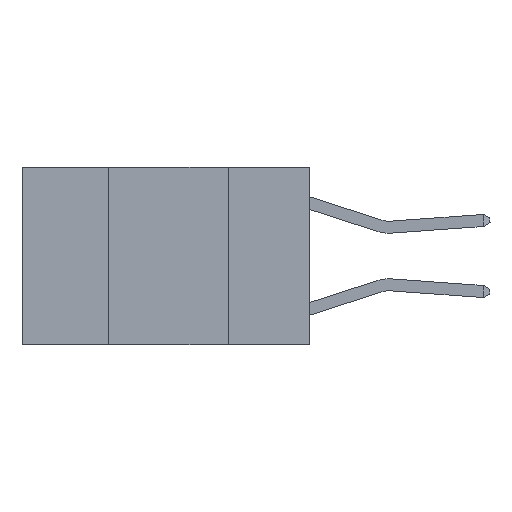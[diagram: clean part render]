
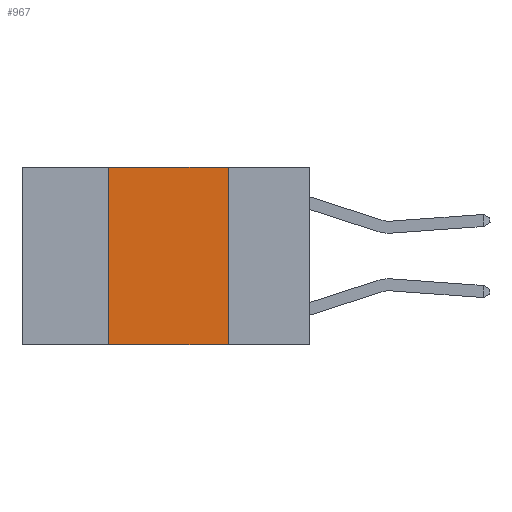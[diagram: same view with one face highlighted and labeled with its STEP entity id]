
A CAD part, left-side view. The second image highlights one B-rep face of the part: STEP entity #967.
In plain terms, the highlighted planar face has unit normal (-1, 0, 0).
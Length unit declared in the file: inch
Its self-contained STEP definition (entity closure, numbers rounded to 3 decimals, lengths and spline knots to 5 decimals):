
#78 = ORIENTED_EDGE ( 'NONE', *, *, #5642, .F. ) ;
#271 = ORIENTED_EDGE ( 'NONE', *, *, #17563, .F. ) ;
#313 = ORIENTED_EDGE ( 'NONE', *, *, #11521, .F. ) ;
#607 = PLANE ( 'NONE',  #19080 ) ;
#947 = ORIENTED_EDGE ( 'NONE', *, *, #10591, .T. ) ;
#967 = ADVANCED_FACE ( 'NONE', ( #11820 ), #607, .F. ) ;
#1670 = VERTEX_POINT ( 'NONE', #7644 ) ;
#1758 = CARTESIAN_POINT ( 'NONE',  ( 0., 0.42, -0.37 ) ) ;
#2449 = VECTOR ( 'NONE', #8322, 39.37008 ) ;
#2962 = VERTEX_POINT ( 'NONE', #1758 ) ;
#5642 = EDGE_CURVE ( 'NONE', #1670, #18077, #13989, .T. ) ;
#6586 = DIRECTION ( 'NONE',  ( 0., 0., -1. ) ) ;
#7082 = CARTESIAN_POINT ( 'NONE',  ( 0., 0.42, 0. ) ) ;
#7644 = CARTESIAN_POINT ( 'NONE',  ( 0., 0.17, 0. ) ) ;
#7952 = DIRECTION ( 'NONE',  ( 0., -1., 0. ) ) ;
#8322 = DIRECTION ( 'NONE',  ( 0., 0., -1. ) ) ;
#8584 = DIRECTION ( 'NONE',  ( 0., 0., 1. ) ) ;
#9058 = VECTOR ( 'NONE', #7952, 39.37008 ) ;
#9167 = VECTOR ( 'NONE', #15665, 39.37008 ) ;
#9827 = VERTEX_POINT ( 'NONE', #19025 ) ;
#10449 = DIRECTION ( 'NONE',  ( 1., 0., 0. ) ) ;
#10591 = EDGE_CURVE ( 'NONE', #2962, #18077, #17061, .T. ) ;
#11521 = EDGE_CURVE ( 'NONE', #2962, #9827, #14922, .T. ) ;
#11820 = FACE_OUTER_BOUND ( 'NONE', #14012, .T. ) ;
#12239 = CARTESIAN_POINT ( 'NONE',  ( 0., 0.17, -0.37 ) ) ;
#12422 = CARTESIAN_POINT ( 'NONE',  ( 0., 0.6, -0.37 ) ) ;
#13151 = LINE ( 'NONE', #18550, #9167 ) ;
#13989 = LINE ( 'NONE', #18808, #2449 ) ;
#14012 = EDGE_LOOP ( 'NONE', ( #78, #271, #313, #947 ) ) ;
#14447 = VECTOR ( 'NONE', #8584, 39.37008 ) ;
#14922 = LINE ( 'NONE', #7082, #14447 ) ;
#15665 = DIRECTION ( 'NONE',  ( 0., -1., 0. ) ) ;
#17061 = LINE ( 'NONE', #12422, #9058 ) ;
#17563 = EDGE_CURVE ( 'NONE', #9827, #1670, #13151, .T. ) ;
#18077 = VERTEX_POINT ( 'NONE', #12239 ) ;
#18550 = CARTESIAN_POINT ( 'NONE',  ( 0., 0.6, 0. ) ) ;
#18808 = CARTESIAN_POINT ( 'NONE',  ( 0., 0.17, 0. ) ) ;
#19025 = CARTESIAN_POINT ( 'NONE',  ( 0., 0.42, 0. ) ) ;
#19080 = AXIS2_PLACEMENT_3D ( 'NONE', #19190, #10449, #6586 ) ;
#19190 = CARTESIAN_POINT ( 'NONE',  ( 0., 0.6, 0. ) ) ;
